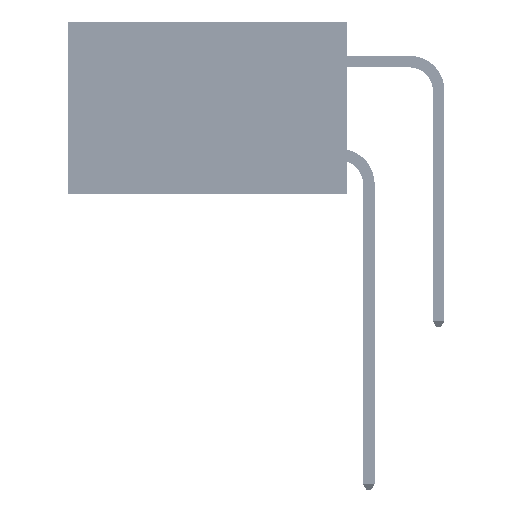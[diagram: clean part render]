
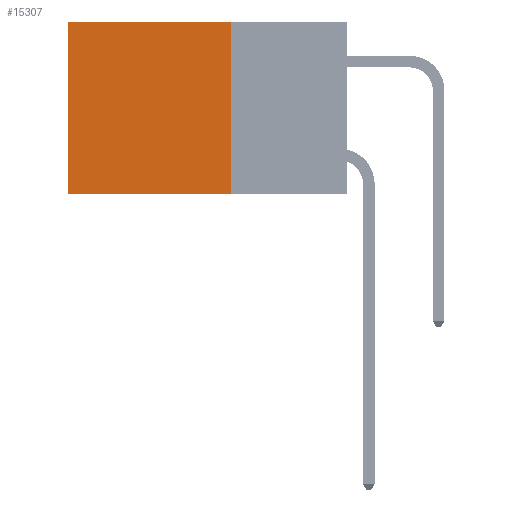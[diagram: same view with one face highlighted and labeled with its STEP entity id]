
A CAD part, left-side view. The second image highlights one B-rep face of the part: STEP entity #15307.
In plain terms, the highlighted planar face has unit normal (-1, 0, 0).
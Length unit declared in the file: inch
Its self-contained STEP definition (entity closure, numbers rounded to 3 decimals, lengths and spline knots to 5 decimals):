
#441 = DIRECTION ( 'NONE',  ( 0., 0., -1. ) ) ;
#1514 = VERTEX_POINT ( 'NONE', #20134 ) ;
#2274 = DIRECTION ( 'NONE',  ( 0., 0., -1. ) ) ;
#7083 = LINE ( 'NONE', #8359, #23453 ) ;
#8012 = LINE ( 'NONE', #45977, #46411 ) ;
#8359 = CARTESIAN_POINT ( 'NONE',  ( 0.2875, 0.25, 0. ) ) ;
#9853 = CARTESIAN_POINT ( 'NONE',  ( 0.2875, 0.6, -0.37 ) ) ;
#10895 = DIRECTION ( 'NONE',  ( 1., 0., 0. ) ) ;
#15307 = ADVANCED_FACE ( 'NONE', ( #29149 ), #38865, .F. ) ;
#18194 = ORIENTED_EDGE ( 'NONE', *, *, #39366, .T. ) ;
#18674 = ORIENTED_EDGE ( 'NONE', *, *, #37461, .F. ) ;
#18964 = EDGE_CURVE ( 'NONE', #24716, #20313, #8012, .T. ) ;
#19426 = DIRECTION ( 'NONE',  ( 0., 1., 0. ) ) ;
#19736 = ORIENTED_EDGE ( 'NONE', *, *, #18964, .T. ) ;
#20134 = CARTESIAN_POINT ( 'NONE',  ( 0.2875, 0.25, 0. ) ) ;
#20313 = VERTEX_POINT ( 'NONE', #9853 ) ;
#23420 = CARTESIAN_POINT ( 'NONE',  ( 0.2875, 0.25, 0. ) ) ;
#23453 = VECTOR ( 'NONE', #441, 39.37008 ) ;
#24716 = VERTEX_POINT ( 'NONE', #46230 ) ;
#25180 = LINE ( 'NONE', #23420, #42175 ) ;
#26945 = CARTESIAN_POINT ( 'NONE',  ( 0.2875, 0.25, -0.37 ) ) ;
#29149 = FACE_OUTER_BOUND ( 'NONE', #39002, .T. ) ;
#31139 = ORIENTED_EDGE ( 'NONE', *, *, #44051, .F. ) ;
#34655 = CARTESIAN_POINT ( 'NONE',  ( 0.2875, 0.25, 0. ) ) ;
#36641 = AXIS2_PLACEMENT_3D ( 'NONE', #34655, #10895, #2274 ) ;
#37461 = EDGE_CURVE ( 'NONE', #1514, #39337, #7083, .T. ) ;
#37971 = VECTOR ( 'NONE', #19426, 39.37008 ) ;
#38865 = PLANE ( 'NONE',  #36641 ) ;
#39002 = EDGE_LOOP ( 'NONE', ( #19736, #31139, #18674, #18194 ) ) ;
#39337 = VERTEX_POINT ( 'NONE', #51866 ) ;
#39366 = EDGE_CURVE ( 'NONE', #1514, #24716, #25180, .T. ) ;
#40551 = DIRECTION ( 'NONE',  ( 0., 0., -1. ) ) ;
#42175 = VECTOR ( 'NONE', #52048, 39.37008 ) ;
#44051 = EDGE_CURVE ( 'NONE', #39337, #20313, #51791, .T. ) ;
#45977 = CARTESIAN_POINT ( 'NONE',  ( 0.2875, 0.6, 0. ) ) ;
#46230 = CARTESIAN_POINT ( 'NONE',  ( 0.2875, 0.6, 0. ) ) ;
#46411 = VECTOR ( 'NONE', #40551, 39.37008 ) ;
#51791 = LINE ( 'NONE', #26945, #37971 ) ;
#51866 = CARTESIAN_POINT ( 'NONE',  ( 0.2875, 0.25, -0.37 ) ) ;
#52048 = DIRECTION ( 'NONE',  ( 0., 1., 0. ) ) ;
